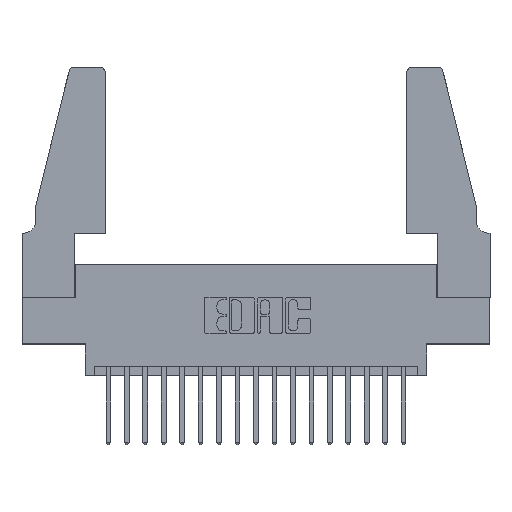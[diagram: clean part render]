
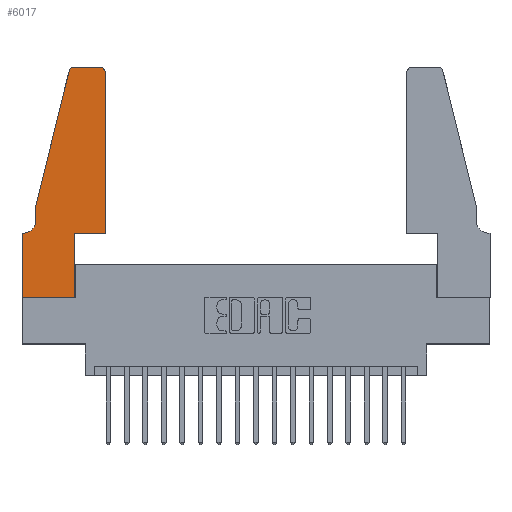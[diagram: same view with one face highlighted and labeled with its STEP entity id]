
A CAD part, top view. The second image highlights one B-rep face of the part: STEP entity #6017.
In plain terms, the highlighted planar face has unit normal (0, 0, 1).
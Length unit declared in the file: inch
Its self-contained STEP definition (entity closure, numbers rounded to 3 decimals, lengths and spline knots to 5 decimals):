
#113 = VERTEX_POINT ( 'NONE', #17261 ) ;
#735 = CARTESIAN_POINT ( 'NONE',  ( 0.0755, 0.5, 0.37 ) ) ;
#816 = VECTOR ( 'NONE', #9589, 39.37008 ) ;
#849 = LINE ( 'NONE', #15923, #1728 ) ;
#952 = CARTESIAN_POINT ( 'NONE',  ( 0.0755, 0.35, 0.37 ) ) ;
#961 = CARTESIAN_POINT ( 'NONE',  ( 0., 0., 0.37 ) ) ;
#1044 = DIRECTION ( 'NONE',  ( -1., 0., 0. ) ) ;
#1238 = VECTOR ( 'NONE', #16904, 39.37008 ) ;
#1289 = VECTOR ( 'NONE', #12387, 39.37008 ) ;
#1314 = EDGE_LOOP ( 'NONE', ( #16579, #14810, #17836, #12738, #15984, #14462, #5468, #18429, #5661, #15824, #3000, #18092 ) ) ;
#1374 = CARTESIAN_POINT ( 'NONE',  ( 0.0055, 0.35, 0.37 ) ) ;
#1676 = DIRECTION ( 'NONE',  ( 0., 0., 1. ) ) ;
#1728 = VECTOR ( 'NONE', #7179, 39.37008 ) ;
#1969 = CARTESIAN_POINT ( 'NONE',  ( 0.2865, 0.35, 0.37 ) ) ;
#2455 = VERTEX_POINT ( 'NONE', #6443 ) ;
#3000 = ORIENTED_EDGE ( 'NONE', *, *, #7619, .T. ) ;
#3290 = VECTOR ( 'NONE', #17230, 39.37008 ) ;
#3373 = VERTEX_POINT ( 'NONE', #735 ) ;
#3838 = VECTOR ( 'NONE', #16721, 39.37008 ) ;
#3853 = CARTESIAN_POINT ( 'NONE',  ( 0., 0., 0.37 ) ) ;
#4233 = VERTEX_POINT ( 'NONE', #3853 ) ;
#5213 = LINE ( 'NONE', #17991, #1289 ) ;
#5468 = ORIENTED_EDGE ( 'NONE', *, *, #14602, .T. ) ;
#5605 = EDGE_CURVE ( 'NONE', #14179, #7566, #5213, .T. ) ;
#5632 = LINE ( 'NONE', #18513, #1238 ) ;
#5656 = EDGE_CURVE ( 'NONE', #9403, #14179, #11568, .T. ) ;
#5661 = ORIENTED_EDGE ( 'NONE', *, *, #5656, .T. ) ;
#5694 = EDGE_CURVE ( 'NONE', #3373, #13545, #10632, .T. ) ;
#5942 = VECTOR ( 'NONE', #17895, 39.37008 ) ;
#6017 = ADVANCED_FACE ( 'NONE', ( #11551 ), #15087, .T. ) ;
#6424 = CARTESIAN_POINT ( 'NONE',  ( 0., 0.35, 0.37 ) ) ;
#6443 = CARTESIAN_POINT ( 'NONE',  ( 0., 0.35, 0.37 ) ) ;
#6785 = DIRECTION ( 'NONE',  ( 0., 0., -1. ) ) ;
#6789 = CARTESIAN_POINT ( 'NONE',  ( 0.284, 1.25, 0.37 ) ) ;
#6834 = CIRCLE ( 'NONE', #19006, 0.03 ) ;
#7034 = CIRCLE ( 'NONE', #14776, 0.07 ) ;
#7179 = DIRECTION ( 'NONE',  ( -0.239, -0.971, 0. ) ) ;
#7566 = VERTEX_POINT ( 'NONE', #12702 ) ;
#7619 = EDGE_CURVE ( 'NONE', #7566, #8707, #5632, .T. ) ;
#7674 = EDGE_CURVE ( 'NONE', #11361, #2455, #14291, .T. ) ;
#8084 = DIRECTION ( 'NONE',  ( 1., 0., 0. ) ) ;
#8356 = EDGE_CURVE ( 'NONE', #18947, #18979, #10127, .T. ) ;
#8512 = CARTESIAN_POINT ( 'NONE',  ( 0.0755, 0.42, 0.37 ) ) ;
#8707 = VERTEX_POINT ( 'NONE', #11684 ) ;
#9403 = VERTEX_POINT ( 'NONE', #12088 ) ;
#9589 = DIRECTION ( 'NONE',  ( 0., -1., 0. ) ) ;
#9695 = DIRECTION ( 'NONE',  ( 1., 0., 0. ) ) ;
#9890 = DIRECTION ( 'NONE',  ( 0., 0., 1. ) ) ;
#10078 = CARTESIAN_POINT ( 'NONE',  ( 0.4205, 1.22, 0.37 ) ) ;
#10127 = CIRCLE ( 'NONE', #18662, 0.03 ) ;
#10632 = LINE ( 'NONE', #15556, #816 ) ;
#10649 = CARTESIAN_POINT ( 'NONE',  ( 0.25487, 1.22718, 0.37 ) ) ;
#10909 = LINE ( 'NONE', #13335, #5942 ) ;
#11293 = LINE ( 'NONE', #11886, #14100 ) ;
#11361 = VERTEX_POINT ( 'NONE', #1374 ) ;
#11380 = VECTOR ( 'NONE', #8084, 39.37008 ) ;
#11551 = FACE_OUTER_BOUND ( 'NONE', #1314, .T. ) ;
#11568 = LINE ( 'NONE', #1969, #3838 ) ;
#11684 = CARTESIAN_POINT ( 'NONE',  ( 0.4505, 1.22, 0.37 ) ) ;
#11886 = CARTESIAN_POINT ( 'NONE',  ( 0.2605, 1.25, 0.37 ) ) ;
#11902 = DIRECTION ( 'NONE',  ( 1., 0., 0. ) ) ;
#12088 = CARTESIAN_POINT ( 'NONE',  ( 0.2865, 0., 0.37 ) ) ;
#12130 = AXIS2_PLACEMENT_3D ( 'NONE', #6424, #1676, #11902 ) ;
#12387 = DIRECTION ( 'NONE',  ( 1., 0., 0. ) ) ;
#12702 = CARTESIAN_POINT ( 'NONE',  ( 0.4505, 0.35, 0.37 ) ) ;
#12738 = ORIENTED_EDGE ( 'NONE', *, *, #5694, .T. ) ;
#13019 = DIRECTION ( 'NONE',  ( 1., 0., 0. ) ) ;
#13335 = CARTESIAN_POINT ( 'NONE',  ( 0., 0., 0.37 ) ) ;
#13545 = VERTEX_POINT ( 'NONE', #8512 ) ;
#14100 = VECTOR ( 'NONE', #16159, 39.37008 ) ;
#14123 = CARTESIAN_POINT ( 'NONE',  ( 0.0055, 0.42, 0.37 ) ) ;
#14179 = VERTEX_POINT ( 'NONE', #18610 ) ;
#14257 = DIRECTION ( 'NONE',  ( 0., 0., 1. ) ) ;
#14291 = LINE ( 'NONE', #952, #3290 ) ;
#14462 = ORIENTED_EDGE ( 'NONE', *, *, #7674, .T. ) ;
#14602 = EDGE_CURVE ( 'NONE', #2455, #4233, #10909, .T. ) ;
#14776 = AXIS2_PLACEMENT_3D ( 'NONE', #14123, #6785, #1044 ) ;
#14810 = ORIENTED_EDGE ( 'NONE', *, *, #8356, .T. ) ;
#14873 = EDGE_CURVE ( 'NONE', #18979, #3373, #849, .T. ) ;
#15087 = PLANE ( 'NONE',  #12130 ) ;
#15311 = LINE ( 'NONE', #961, #11380 ) ;
#15556 = CARTESIAN_POINT ( 'NONE',  ( 0.0755, 0.5, 0.37 ) ) ;
#15604 = EDGE_CURVE ( 'NONE', #13545, #11361, #7034, .T. ) ;
#15824 = ORIENTED_EDGE ( 'NONE', *, *, #5605, .T. ) ;
#15923 = CARTESIAN_POINT ( 'NONE',  ( 0.0755, 0.5, 0.37 ) ) ;
#15984 = ORIENTED_EDGE ( 'NONE', *, *, #15604, .T. ) ;
#16159 = DIRECTION ( 'NONE',  ( -1., 0., 0. ) ) ;
#16363 = EDGE_CURVE ( 'NONE', #113, #18947, #11293, .T. ) ;
#16579 = ORIENTED_EDGE ( 'NONE', *, *, #16363, .T. ) ;
#16721 = DIRECTION ( 'NONE',  ( 0., 1., 0. ) ) ;
#16904 = DIRECTION ( 'NONE',  ( 0., 1., 0. ) ) ;
#17026 = CARTESIAN_POINT ( 'NONE',  ( 0.284, 1.22, 0.37 ) ) ;
#17230 = DIRECTION ( 'NONE',  ( -1., 0., 0. ) ) ;
#17261 = CARTESIAN_POINT ( 'NONE',  ( 0.4205, 1.25, 0.37 ) ) ;
#17731 = EDGE_CURVE ( 'NONE', #4233, #9403, #15311, .T. ) ;
#17836 = ORIENTED_EDGE ( 'NONE', *, *, #14873, .T. ) ;
#17895 = DIRECTION ( 'NONE',  ( 0., -1., 0. ) ) ;
#17991 = CARTESIAN_POINT ( 'NONE',  ( 0.4505, 0.35, 0.37 ) ) ;
#18092 = ORIENTED_EDGE ( 'NONE', *, *, #18375, .T. ) ;
#18375 = EDGE_CURVE ( 'NONE', #8707, #113, #6834, .T. ) ;
#18429 = ORIENTED_EDGE ( 'NONE', *, *, #17731, .T. ) ;
#18513 = CARTESIAN_POINT ( 'NONE',  ( 0.4505, 0.35, 0.37 ) ) ;
#18610 = CARTESIAN_POINT ( 'NONE',  ( 0.2865, 0.35, 0.37 ) ) ;
#18662 = AXIS2_PLACEMENT_3D ( 'NONE', #17026, #14257, #9695 ) ;
#18947 = VERTEX_POINT ( 'NONE', #6789 ) ;
#18979 = VERTEX_POINT ( 'NONE', #10649 ) ;
#19006 = AXIS2_PLACEMENT_3D ( 'NONE', #10078, #9890, #13019 ) ;
